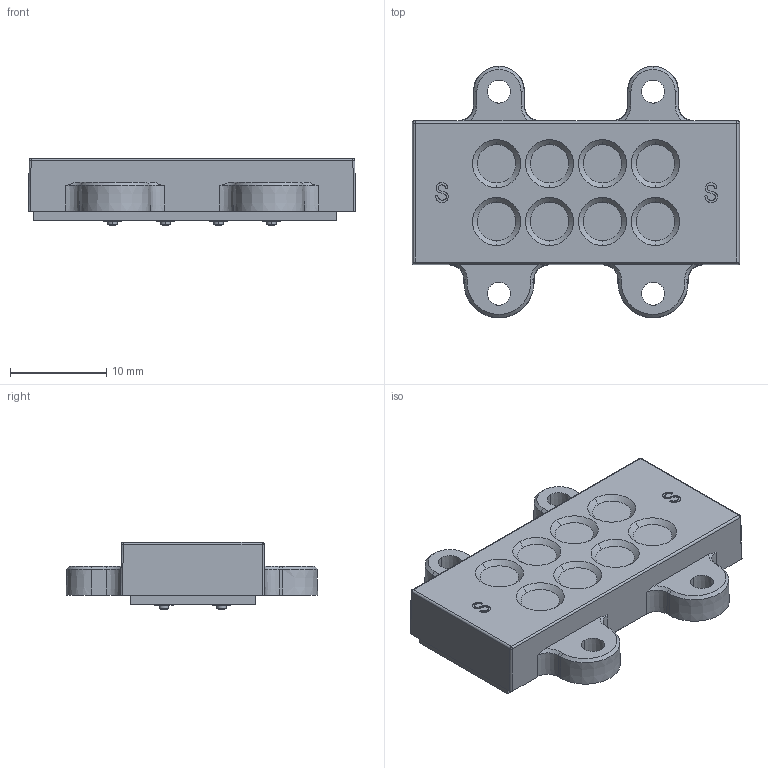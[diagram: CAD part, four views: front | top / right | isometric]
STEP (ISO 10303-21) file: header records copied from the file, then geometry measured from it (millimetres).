
FILE_DESCRIPTION (( 'STEP AP203' ), '1' );
FILE_NAME ('686A0811220113E.STEP', '2023-03-02T06:00:13', ( 'Magnum' ), ( '' ), 'SwSTEP 2.0', 'SolidWorks 2020', '' );
FILE_SCHEMA (( 'CONFIG_CONTROL_DESIGN' ));
Length unit declared in the file: millimetre
Products named in the file (1): 686A0811220113E
Bounding box: 34 x 26.15 x 7 mm (x, y, z)
Volume: 2993.5 mm3; surface area: 3749.5 mm2
Topology: 1 solids, 22 shells, 459 faces, 1065 edges, 694 vertices
Faces by surface type: plane 200, cylinder 155, cone 68, bspline 32, sphere 4
Entity records: 14960 total; most frequent: CARTESIAN_POINT 4233, DIRECTION 2255, ORIENTED_EDGE 2130, EDGE_CURVE 1065, AXIS2_PLACEMENT_3D 840, VERTEX_POINT 694, LINE 575, VECTOR 575
